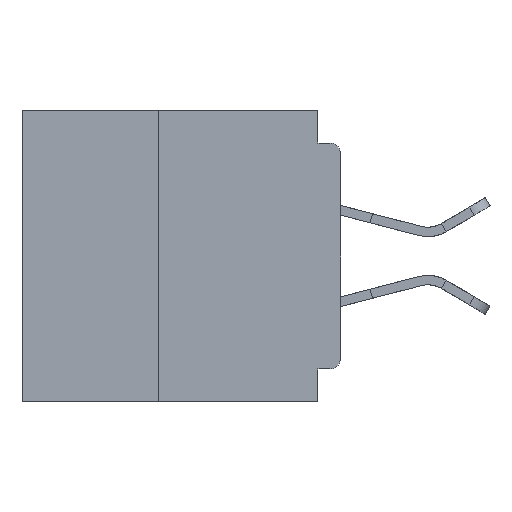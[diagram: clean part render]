
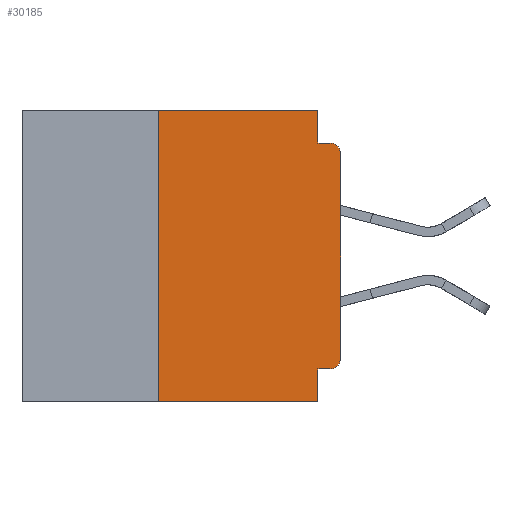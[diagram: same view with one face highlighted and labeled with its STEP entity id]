
A CAD part, left-side view. The second image highlights one B-rep face of the part: STEP entity #30185.
In plain terms, the highlighted planar face has unit normal (-1, 0, 0).
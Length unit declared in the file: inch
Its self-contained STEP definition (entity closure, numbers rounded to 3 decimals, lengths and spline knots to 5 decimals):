
#295 = CARTESIAN_POINT ( 'NONE',  ( 0., 0.031, -0.355 ) ) ;
#920 = CARTESIAN_POINT ( 'NONE',  ( 0., 0.015, -0.06 ) ) ;
#1532 = ORIENTED_EDGE ( 'NONE', *, *, #33820, .T. ) ;
#2431 = CARTESIAN_POINT ( 'NONE',  ( 0., 0., -0.355 ) ) ;
#2703 = AXIS2_PLACEMENT_3D ( 'NONE', #920, #27587, #4746 ) ;
#2739 = CARTESIAN_POINT ( 'NONE',  ( 0., 0.015, -0.34 ) ) ;
#2747 = VERTEX_POINT ( 'NONE', #20653 ) ;
#2975 = LINE ( 'NONE', #30680, #42220 ) ;
#3170 = VERTEX_POINT ( 'NONE', #7119 ) ;
#3798 = DIRECTION ( 'NONE',  ( 0., 0., -1. ) ) ;
#4115 = VERTEX_POINT ( 'NONE', #295 ) ;
#4746 = DIRECTION ( 'NONE',  ( 0., 0., -1. ) ) ;
#4881 = VERTEX_POINT ( 'NONE', #17059 ) ;
#5835 = CARTESIAN_POINT ( 'NONE',  ( 0., 0., -0.045 ) ) ;
#5852 = LINE ( 'NONE', #2431, #33878 ) ;
#6565 = DIRECTION ( 'NONE',  ( 0., 0., -1. ) ) ;
#7119 = CARTESIAN_POINT ( 'NONE',  ( 0., 0.25, 0. ) ) ;
#7540 = VECTOR ( 'NONE', #9897, 39.37008 ) ;
#8918 = VECTOR ( 'NONE', #34197, 39.37008 ) ;
#9186 = ORIENTED_EDGE ( 'NONE', *, *, #47552, .T. ) ;
#9802 = ORIENTED_EDGE ( 'NONE', *, *, #34691, .F. ) ;
#9897 = DIRECTION ( 'NONE',  ( 0., 0., 1. ) ) ;
#10423 = CARTESIAN_POINT ( 'NONE',  ( 0., 0.015, -0.045 ) ) ;
#10485 = VERTEX_POINT ( 'NONE', #34820 ) ;
#11157 = CARTESIAN_POINT ( 'NONE',  ( 0., 0., 0. ) ) ;
#11424 = EDGE_CURVE ( 'NONE', #2747, #4115, #5852, .T. ) ;
#12753 = ORIENTED_EDGE ( 'NONE', *, *, #34366, .F. ) ;
#12911 = AXIS2_PLACEMENT_3D ( 'NONE', #43618, #36226, #13345 ) ;
#13345 = DIRECTION ( 'NONE',  ( 0., 0., -1. ) ) ;
#13374 = ORIENTED_EDGE ( 'NONE', *, *, #28443, .F. ) ;
#14255 = CARTESIAN_POINT ( 'NONE',  ( 0., 0.437, -0.4 ) ) ;
#16924 = CARTESIAN_POINT ( 'NONE',  ( 0., 0., -0.06 ) ) ;
#16998 = ORIENTED_EDGE ( 'NONE', *, *, #28069, .F. ) ;
#17059 = CARTESIAN_POINT ( 'NONE',  ( 0., 0., -0.34 ) ) ;
#17683 = LINE ( 'NONE', #36581, #7540 ) ;
#19135 = CARTESIAN_POINT ( 'NONE',  ( 0., 0.031, -0.4 ) ) ;
#19779 = VERTEX_POINT ( 'NONE', #32301 ) ;
#20246 = EDGE_CURVE ( 'NONE', #3170, #46080, #30105, .T. ) ;
#20653 = CARTESIAN_POINT ( 'NONE',  ( 0., 0.015, -0.355 ) ) ;
#21790 = DIRECTION ( 'NONE',  ( 0., -1., 0. ) ) ;
#24847 = DIRECTION ( 'NONE',  ( 0., -1., 0. ) ) ;
#25159 = EDGE_LOOP ( 'NONE', ( #34828, #9186, #12753, #9802, #42547, #13374, #43721, #16998, #30766, #1532 ) ) ;
#27454 = VECTOR ( 'NONE', #24847, 39.37008 ) ;
#27478 = VECTOR ( 'NONE', #21790, 39.37008 ) ;
#27587 = DIRECTION ( 'NONE',  ( -1., 0., 0. ) ) ;
#28069 = EDGE_CURVE ( 'NONE', #4115, #19779, #44911, .T. ) ;
#28443 = EDGE_CURVE ( 'NONE', #43403, #3170, #17683, .T. ) ;
#29239 = LINE ( 'NONE', #11157, #8918 ) ;
#29425 = DIRECTION ( 'NONE',  ( -1., 0., 0. ) ) ;
#30105 = LINE ( 'NONE', #42469, #37782 ) ;
#30185 = ADVANCED_FACE ( 'NONE', ( #33624 ), #32423, .F. ) ;
#30365 = CIRCLE ( 'NONE', #2703, 0.015 ) ;
#30680 = CARTESIAN_POINT ( 'NONE',  ( 0., 0.031, 0. ) ) ;
#30766 = ORIENTED_EDGE ( 'NONE', *, *, #11424, .F. ) ;
#32255 = EDGE_CURVE ( 'NONE', #4881, #43857, #29239, .T. ) ;
#32301 = CARTESIAN_POINT ( 'NONE',  ( 0., 0.031, -0.4 ) ) ;
#32302 = CIRCLE ( 'NONE', #35472, 0.015 ) ;
#32423 = PLANE ( 'NONE',  #12911 ) ;
#32812 = CARTESIAN_POINT ( 'NONE',  ( 0., 0.25, -0.4 ) ) ;
#33204 = VERTEX_POINT ( 'NONE', #10423 ) ;
#33624 = FACE_OUTER_BOUND ( 'NONE', #25159, .T. ) ;
#33820 = EDGE_CURVE ( 'NONE', #2747, #4881, #32302, .T. ) ;
#33878 = VECTOR ( 'NONE', #40537, 39.37008 ) ;
#34197 = DIRECTION ( 'NONE',  ( 0., 0., 1. ) ) ;
#34366 = EDGE_CURVE ( 'NONE', #10485, #33204, #38746, .T. ) ;
#34458 = DIRECTION ( 'NONE',  ( 0., 0., -1. ) ) ;
#34691 = EDGE_CURVE ( 'NONE', #46080, #10485, #2975, .T. ) ;
#34820 = CARTESIAN_POINT ( 'NONE',  ( 0., 0.031, -0.045 ) ) ;
#34828 = ORIENTED_EDGE ( 'NONE', *, *, #32255, .T. ) ;
#35472 = AXIS2_PLACEMENT_3D ( 'NONE', #2739, #29425, #6565 ) ;
#36226 = DIRECTION ( 'NONE',  ( 1., 0., 0. ) ) ;
#36581 = CARTESIAN_POINT ( 'NONE',  ( 0., 0.25, -0.4 ) ) ;
#37782 = VECTOR ( 'NONE', #46383, 39.37008 ) ;
#38746 = LINE ( 'NONE', #5835, #27454 ) ;
#40537 = DIRECTION ( 'NONE',  ( 0., 1., 0. ) ) ;
#41873 = CARTESIAN_POINT ( 'NONE',  ( 0., 0.031, 0. ) ) ;
#42220 = VECTOR ( 'NONE', #34458, 39.37008 ) ;
#42469 = CARTESIAN_POINT ( 'NONE',  ( 0., 0.437, 0. ) ) ;
#42547 = ORIENTED_EDGE ( 'NONE', *, *, #20246, .F. ) ;
#43403 = VERTEX_POINT ( 'NONE', #32812 ) ;
#43497 = EDGE_CURVE ( 'NONE', #43403, #19779, #48696, .T. ) ;
#43618 = CARTESIAN_POINT ( 'NONE',  ( 0., 0.437, 0. ) ) ;
#43721 = ORIENTED_EDGE ( 'NONE', *, *, #43497, .T. ) ;
#43771 = VECTOR ( 'NONE', #3798, 39.37008 ) ;
#43857 = VERTEX_POINT ( 'NONE', #16924 ) ;
#44911 = LINE ( 'NONE', #19135, #43771 ) ;
#46080 = VERTEX_POINT ( 'NONE', #41873 ) ;
#46383 = DIRECTION ( 'NONE',  ( 0., -1., 0. ) ) ;
#47552 = EDGE_CURVE ( 'NONE', #43857, #33204, #30365, .T. ) ;
#48696 = LINE ( 'NONE', #14255, #27478 ) ;
